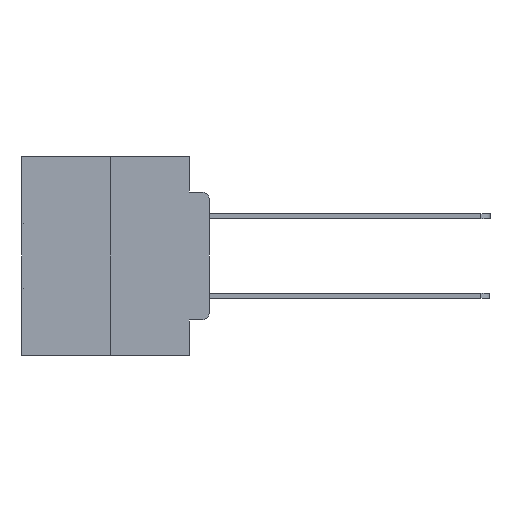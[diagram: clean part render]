
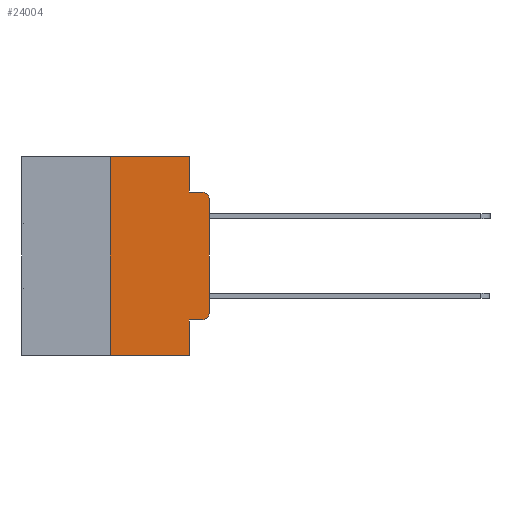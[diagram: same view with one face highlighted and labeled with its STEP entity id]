
A CAD part, left-side view. The second image highlights one B-rep face of the part: STEP entity #24004.
In plain terms, the highlighted planar face has unit normal (-1, 0, 0).
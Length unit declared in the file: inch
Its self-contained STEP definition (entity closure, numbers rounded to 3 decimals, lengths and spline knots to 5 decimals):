
#266 = EDGE_CURVE ( 'NONE', #24088, #3499, #20107, .T. ) ;
#424 = DIRECTION ( 'NONE',  ( 0., -1., 0. ) ) ;
#592 = DIRECTION ( 'NONE',  ( 0., -1., 0. ) ) ;
#958 = VECTOR ( 'NONE', #424, 39.37008 ) ;
#1143 = VERTEX_POINT ( 'NONE', #24686 ) ;
#1183 = CARTESIAN_POINT ( 'NONE',  ( 0., 0.02, -0.1085 ) ) ;
#1324 = ORIENTED_EDGE ( 'NONE', *, *, #21689, .T. ) ;
#1541 = ORIENTED_EDGE ( 'NONE', *, *, #29784, .F. ) ;
#1607 = VECTOR ( 'NONE', #20822, 39.37008 ) ;
#1966 = ORIENTED_EDGE ( 'NONE', *, *, #10688, .F. ) ;
#2069 = DIRECTION ( 'NONE',  ( 0., -1., 0. ) ) ;
#2083 = LINE ( 'NONE', #2972, #13661 ) ;
#2192 = EDGE_LOOP ( 'NONE', ( #9992, #26479, #25428, #1541, #1966, #12043, #1324, #10104, #9230, #19508 ) ) ;
#2307 = VERTEX_POINT ( 'NONE', #24507 ) ;
#2814 = CARTESIAN_POINT ( 'NONE',  ( 0., 0.051, -0.0885 ) ) ;
#2972 = CARTESIAN_POINT ( 'NONE',  ( 0., 0.473, 0. ) ) ;
#3219 = CARTESIAN_POINT ( 'NONE',  ( 0., 0.02, -0.4115 ) ) ;
#3499 = VERTEX_POINT ( 'NONE', #18273 ) ;
#3548 = DIRECTION ( 'NONE',  ( 0., 0., -1. ) ) ;
#4063 = EDGE_CURVE ( 'NONE', #2307, #13743, #18436, .T. ) ;
#6014 = LINE ( 'NONE', #25207, #17555 ) ;
#6170 = VECTOR ( 'NONE', #27663, 39.37008 ) ;
#7218 = LINE ( 'NONE', #28240, #958 ) ;
#7426 = FACE_OUTER_BOUND ( 'NONE', #2192, .T. ) ;
#8143 = CARTESIAN_POINT ( 'NONE',  ( 0., 0.473, -0.5 ) ) ;
#8163 = LINE ( 'NONE', #18408, #19715 ) ;
#8280 = LINE ( 'NONE', #8143, #19841 ) ;
#8674 = AXIS2_PLACEMENT_3D ( 'NONE', #9719, #25971, #12028 ) ;
#9184 = DIRECTION ( 'NONE',  ( 0., 0., 1. ) ) ;
#9230 = ORIENTED_EDGE ( 'NONE', *, *, #12328, .T. ) ;
#9719 = CARTESIAN_POINT ( 'NONE',  ( 0., 0.473, 0. ) ) ;
#9992 = ORIENTED_EDGE ( 'NONE', *, *, #17268, .T. ) ;
#10104 = ORIENTED_EDGE ( 'NONE', *, *, #4063, .F. ) ;
#10411 = DIRECTION ( 'NONE',  ( 0., -1., 0. ) ) ;
#10688 = EDGE_CURVE ( 'NONE', #3499, #1143, #2083, .T. ) ;
#10798 = AXIS2_PLACEMENT_3D ( 'NONE', #1183, #17438, #3548 ) ;
#12028 = DIRECTION ( 'NONE',  ( 0., 0., -1. ) ) ;
#12043 = ORIENTED_EDGE ( 'NONE', *, *, #266, .F. ) ;
#12328 = EDGE_CURVE ( 'NONE', #2307, #14361, #20345, .T. ) ;
#12514 = DIRECTION ( 'NONE',  ( -1., 0., 0. ) ) ;
#13661 = VECTOR ( 'NONE', #592, 39.37008 ) ;
#13743 = VERTEX_POINT ( 'NONE', #24151 ) ;
#14361 = VERTEX_POINT ( 'NONE', #3219 ) ;
#14367 = CARTESIAN_POINT ( 'NONE',  ( 0., 0.02, -0.0885 ) ) ;
#16300 = EDGE_CURVE ( 'NONE', #25290, #18114, #22693, .T. ) ;
#17268 = EDGE_CURVE ( 'NONE', #19913, #25290, #8163, .T. ) ;
#17438 = DIRECTION ( 'NONE',  ( -1., 0., 0. ) ) ;
#17555 = VECTOR ( 'NONE', #27509, 39.37008 ) ;
#18114 = VERTEX_POINT ( 'NONE', #14367 ) ;
#18206 = EDGE_CURVE ( 'NONE', #14361, #19913, #19655, .T. ) ;
#18273 = CARTESIAN_POINT ( 'NONE',  ( 0., 0.25, 0. ) ) ;
#18408 = CARTESIAN_POINT ( 'NONE',  ( 0., 0., 0. ) ) ;
#18436 = LINE ( 'NONE', #27494, #6170 ) ;
#19360 = CARTESIAN_POINT ( 'NONE',  ( 0., 0.25, -0.5 ) ) ;
#19508 = ORIENTED_EDGE ( 'NONE', *, *, #18206, .T. ) ;
#19655 = CIRCLE ( 'NONE', #21308, 0.02 ) ;
#19715 = VECTOR ( 'NONE', #9184, 39.37008 ) ;
#19841 = VECTOR ( 'NONE', #10411, 39.37008 ) ;
#19913 = VERTEX_POINT ( 'NONE', #21970 ) ;
#20107 = LINE ( 'NONE', #22010, #1607 ) ;
#20345 = LINE ( 'NONE', #29763, #25805 ) ;
#20822 = DIRECTION ( 'NONE',  ( 0., 0., 1. ) ) ;
#21205 = CARTESIAN_POINT ( 'NONE',  ( 0., 0., -0.1085 ) ) ;
#21272 = PLANE ( 'NONE',  #8674 ) ;
#21308 = AXIS2_PLACEMENT_3D ( 'NONE', #26466, #12514, #28741 ) ;
#21510 = EDGE_CURVE ( 'NONE', #21533, #18114, #7218, .T. ) ;
#21533 = VERTEX_POINT ( 'NONE', #2814 ) ;
#21689 = EDGE_CURVE ( 'NONE', #24088, #13743, #8280, .T. ) ;
#21970 = CARTESIAN_POINT ( 'NONE',  ( 0., 0., -0.3915 ) ) ;
#22010 = CARTESIAN_POINT ( 'NONE',  ( 0., 0.25, 0. ) ) ;
#22693 = CIRCLE ( 'NONE', #10798, 0.02 ) ;
#24004 = ADVANCED_FACE ( 'NONE', ( #7426 ), #21272, .F. ) ;
#24088 = VERTEX_POINT ( 'NONE', #19360 ) ;
#24151 = CARTESIAN_POINT ( 'NONE',  ( 0., 0.051, -0.5 ) ) ;
#24507 = CARTESIAN_POINT ( 'NONE',  ( 0., 0.051, -0.4115 ) ) ;
#24686 = CARTESIAN_POINT ( 'NONE',  ( 0., 0.051, 0. ) ) ;
#25207 = CARTESIAN_POINT ( 'NONE',  ( 0., 0.051, 0. ) ) ;
#25290 = VERTEX_POINT ( 'NONE', #21205 ) ;
#25428 = ORIENTED_EDGE ( 'NONE', *, *, #21510, .F. ) ;
#25805 = VECTOR ( 'NONE', #2069, 39.37008 ) ;
#25971 = DIRECTION ( 'NONE',  ( 1., 0., 0. ) ) ;
#26466 = CARTESIAN_POINT ( 'NONE',  ( 0., 0.02, -0.3915 ) ) ;
#26479 = ORIENTED_EDGE ( 'NONE', *, *, #16300, .T. ) ;
#27494 = CARTESIAN_POINT ( 'NONE',  ( 0., 0.051, 0. ) ) ;
#27509 = DIRECTION ( 'NONE',  ( 0., 0., -1. ) ) ;
#27663 = DIRECTION ( 'NONE',  ( 0., 0., -1. ) ) ;
#28240 = CARTESIAN_POINT ( 'NONE',  ( 0., 0.051, -0.0885 ) ) ;
#28741 = DIRECTION ( 'NONE',  ( 0., 0., -1. ) ) ;
#29763 = CARTESIAN_POINT ( 'NONE',  ( 0., 0.051, -0.4115 ) ) ;
#29784 = EDGE_CURVE ( 'NONE', #1143, #21533, #6014, .T. ) ;
